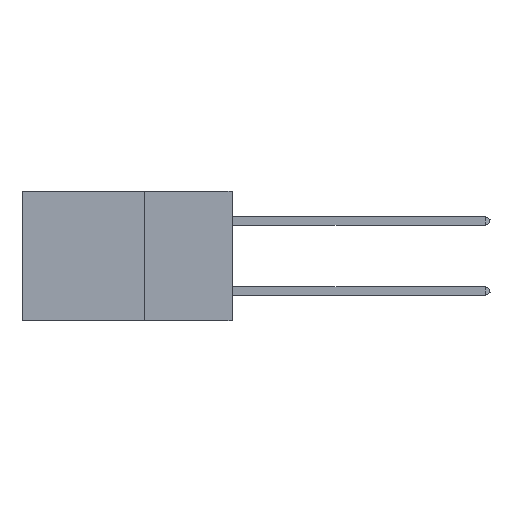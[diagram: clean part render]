
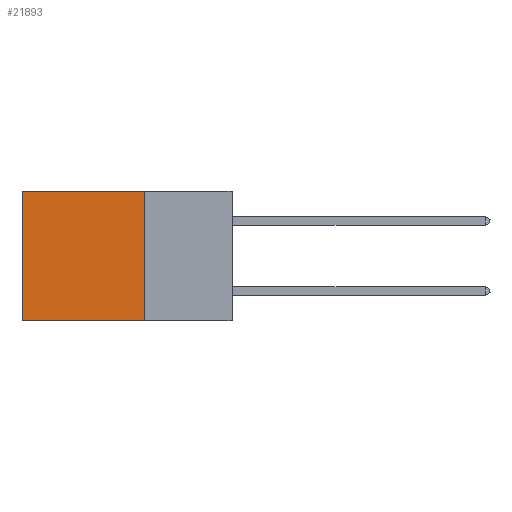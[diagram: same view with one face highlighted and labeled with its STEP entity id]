
A CAD part, left-side view. The second image highlights one B-rep face of the part: STEP entity #21893.
In plain terms, the highlighted planar face has unit normal (-1, 0, 0).
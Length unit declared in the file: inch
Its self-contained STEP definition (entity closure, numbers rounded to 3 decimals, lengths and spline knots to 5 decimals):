
#4656 = CARTESIAN_POINT ( 'NONE',  ( 0.2875, 0.25, 0. ) ) ;
#6063 = FACE_OUTER_BOUND ( 'NONE', #17536, .T. ) ;
#6454 = EDGE_CURVE ( 'NONE', #20366, #27606, #13341, .T. ) ;
#7294 = DIRECTION ( 'NONE',  ( 0., 0., -1. ) ) ;
#7407 = DIRECTION ( 'NONE',  ( 1., 0., 0. ) ) ;
#8024 = VERTEX_POINT ( 'NONE', #34380 ) ;
#8115 = ORIENTED_EDGE ( 'NONE', *, *, #32072, .T. ) ;
#9185 = ORIENTED_EDGE ( 'NONE', *, *, #6454, .T. ) ;
#10207 = PLANE ( 'NONE',  #16618 ) ;
#13341 = LINE ( 'NONE', #24971, #27652 ) ;
#14126 = CARTESIAN_POINT ( 'NONE',  ( 0.2875, 0.25, -0.37 ) ) ;
#14684 = ORIENTED_EDGE ( 'NONE', *, *, #26425, .F. ) ;
#14953 = LINE ( 'NONE', #22781, #24980 ) ;
#15793 = VECTOR ( 'NONE', #19527, 39.37008 ) ;
#16618 = AXIS2_PLACEMENT_3D ( 'NONE', #29292, #7407, #7294 ) ;
#17536 = EDGE_LOOP ( 'NONE', ( #9185, #14684, #34756, #8115 ) ) ;
#19224 = VERTEX_POINT ( 'NONE', #24329 ) ;
#19527 = DIRECTION ( 'NONE',  ( 0., 1., 0. ) ) ;
#19645 = EDGE_CURVE ( 'NONE', #8024, #19224, #28401, .T. ) ;
#20366 = VERTEX_POINT ( 'NONE', #24130 ) ;
#21893 = ADVANCED_FACE ( 'NONE', ( #6063 ), #10207, .F. ) ;
#22781 = CARTESIAN_POINT ( 'NONE',  ( 0.2875, 0.25, 0. ) ) ;
#24130 = CARTESIAN_POINT ( 'NONE',  ( 0.2875, 0.6, 0. ) ) ;
#24329 = CARTESIAN_POINT ( 'NONE',  ( 0.2875, 0.25, -0.37 ) ) ;
#24971 = CARTESIAN_POINT ( 'NONE',  ( 0.2875, 0.6, 0. ) ) ;
#24980 = VECTOR ( 'NONE', #34056, 39.37008 ) ;
#26425 = EDGE_CURVE ( 'NONE', #19224, #27606, #29245, .T. ) ;
#27606 = VERTEX_POINT ( 'NONE', #35297 ) ;
#27652 = VECTOR ( 'NONE', #33629, 39.37008 ) ;
#28401 = LINE ( 'NONE', #4656, #34846 ) ;
#29245 = LINE ( 'NONE', #14126, #15793 ) ;
#29292 = CARTESIAN_POINT ( 'NONE',  ( 0.2875, 0.25, 0. ) ) ;
#32072 = EDGE_CURVE ( 'NONE', #8024, #20366, #14953, .T. ) ;
#33629 = DIRECTION ( 'NONE',  ( 0., 0., -1. ) ) ;
#34056 = DIRECTION ( 'NONE',  ( 0., 1., 0. ) ) ;
#34380 = CARTESIAN_POINT ( 'NONE',  ( 0.2875, 0.25, 0. ) ) ;
#34697 = DIRECTION ( 'NONE',  ( 0., 0., -1. ) ) ;
#34756 = ORIENTED_EDGE ( 'NONE', *, *, #19645, .F. ) ;
#34846 = VECTOR ( 'NONE', #34697, 39.37008 ) ;
#35297 = CARTESIAN_POINT ( 'NONE',  ( 0.2875, 0.6, -0.37 ) ) ;
